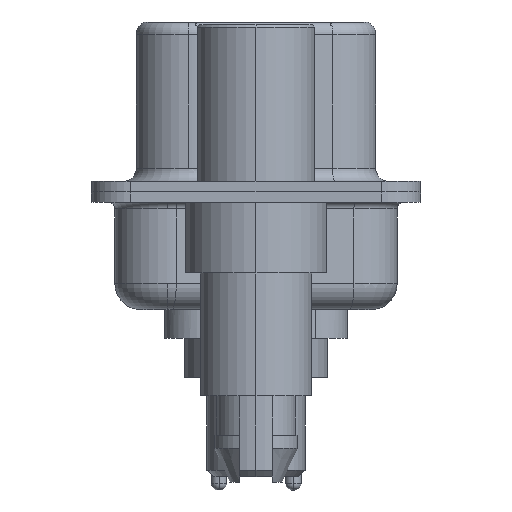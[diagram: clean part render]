
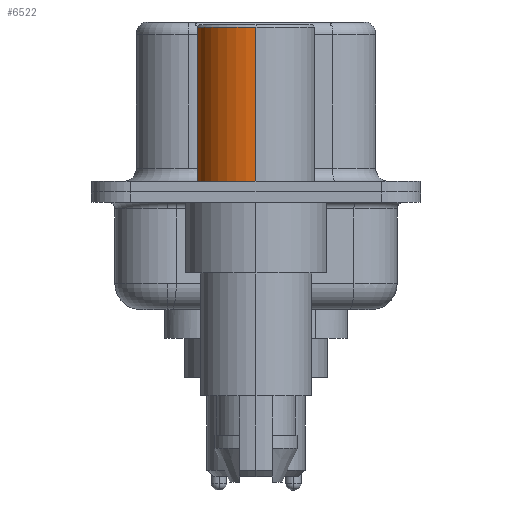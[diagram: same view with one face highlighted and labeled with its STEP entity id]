
A CAD part, left-side view. The second image highlights one B-rep face of the part: STEP entity #6522.
In plain terms, the highlighted cylindrical face has radius 2.25 mm (diameter 4.5 mm), a partial arc.
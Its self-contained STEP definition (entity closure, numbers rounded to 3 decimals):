
#436 = DIRECTION ( 'NONE',  ( 0., 0., 1. ) ) ;
#1851 = AXIS2_PLACEMENT_3D ( 'NONE', #17446, #5403, #19483 ) ;
#2425 = CARTESIAN_POINT ( 'NONE',  ( 0., 0., 6.3 ) ) ;
#2926 = VECTOR ( 'NONE', #436, 1000. ) ;
#3497 = CARTESIAN_POINT ( 'NONE',  ( 2.25, 0., 0.4 ) ) ;
#4468 = LINE ( 'NONE', #8170, #19942 ) ;
#4504 = DIRECTION ( 'NONE',  ( 1., 0., 0. ) ) ;
#4834 = DIRECTION ( 'NONE',  ( 1., 0., 0. ) ) ;
#5403 = DIRECTION ( 'NONE',  ( 0., 0., 1. ) ) ;
#5545 = CIRCLE ( 'NONE', #6923, 2.25 ) ;
#6522 = ADVANCED_FACE ( 'NONE', ( #11160 ), #21200, .T. ) ;
#6923 = AXIS2_PLACEMENT_3D ( 'NONE', #2425, #16581, #4504 ) ;
#7583 = ORIENTED_EDGE ( 'NONE', *, *, #12729, .T. ) ;
#8158 = VERTEX_POINT ( 'NONE', #23449 ) ;
#8170 = CARTESIAN_POINT ( 'NONE',  ( 2.25, 0., 0.581 ) ) ;
#8196 = VERTEX_POINT ( 'NONE', #3497 ) ;
#9679 = LINE ( 'NONE', #12665, #2926 ) ;
#10575 = CARTESIAN_POINT ( 'NONE',  ( 2.25, 0., 6.3 ) ) ;
#11056 = EDGE_CURVE ( 'NONE', #16558, #11914, #5545, .T. ) ;
#11160 = FACE_OUTER_BOUND ( 'NONE', #19019, .T. ) ;
#11914 = VERTEX_POINT ( 'NONE', #12178 ) ;
#12178 = CARTESIAN_POINT ( 'NONE',  ( -2.25, 0., 6.3 ) ) ;
#12665 = CARTESIAN_POINT ( 'NONE',  ( -2.25, 0., 0.581 ) ) ;
#12729 = EDGE_CURVE ( 'NONE', #8158, #11914, #9679, .T. ) ;
#14063 = AXIS2_PLACEMENT_3D ( 'NONE', #14364, #22185, #4834 ) ;
#14364 = CARTESIAN_POINT ( 'NONE',  ( 0., 0., 0.581 ) ) ;
#15236 = EDGE_CURVE ( 'NONE', #8196, #16558, #4468, .T. ) ;
#16558 = VERTEX_POINT ( 'NONE', #10575 ) ;
#16581 = DIRECTION ( 'NONE',  ( 0., 0., 1. ) ) ;
#17446 = CARTESIAN_POINT ( 'NONE',  ( 0., 0., 0.4 ) ) ;
#18128 = DIRECTION ( 'NONE',  ( 0., 0., 1. ) ) ;
#19019 = EDGE_LOOP ( 'NONE', ( #25312, #7583, #24541, #21394 ) ) ;
#19483 = DIRECTION ( 'NONE',  ( 1., 0., 0. ) ) ;
#19942 = VECTOR ( 'NONE', #18128, 1000. ) ;
#21200 = CYLINDRICAL_SURFACE ( 'NONE', #14063, 2.25 ) ;
#21394 = ORIENTED_EDGE ( 'NONE', *, *, #15236, .F. ) ;
#22185 = DIRECTION ( 'NONE',  ( 0., 0., 1. ) ) ;
#23449 = CARTESIAN_POINT ( 'NONE',  ( -2.25, 0., 0.4 ) ) ;
#23991 = EDGE_CURVE ( 'NONE', #8196, #8158, #25835, .T. ) ;
#24541 = ORIENTED_EDGE ( 'NONE', *, *, #11056, .F. ) ;
#25312 = ORIENTED_EDGE ( 'NONE', *, *, #23991, .T. ) ;
#25835 = CIRCLE ( 'NONE', #1851, 2.25 ) ;
